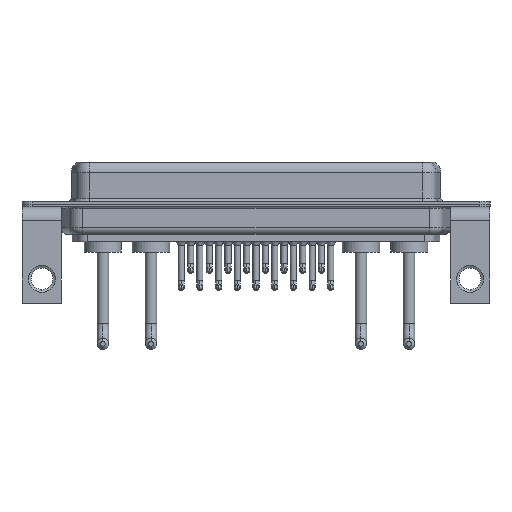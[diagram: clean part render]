
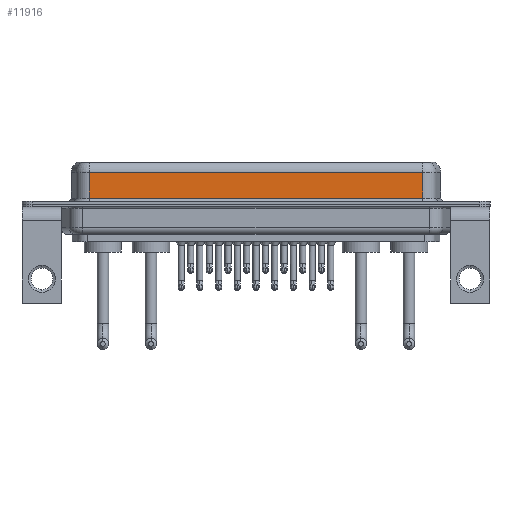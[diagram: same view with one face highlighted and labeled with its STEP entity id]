
A CAD part, front view. The second image highlights one B-rep face of the part: STEP entity #11916.
In plain terms, the highlighted planar face has unit normal (0, -1, 0).
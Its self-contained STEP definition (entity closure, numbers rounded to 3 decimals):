
#147 = EDGE_CURVE ( 'NONE', #21658, #11551, #12469, .T. ) ;
#1646 = CARTESIAN_POINT ( 'NONE',  ( 56.462, -3.95, 6.4 ) ) ;
#1962 = DIRECTION ( 'NONE',  ( 1., 0., 0. ) ) ;
#3037 = LINE ( 'NONE', #1646, #22165 ) ;
#3250 = VERTEX_POINT ( 'NONE', #12139 ) ;
#4416 = ORIENTED_EDGE ( 'NONE', *, *, #4469, .F. ) ;
#4469 = EDGE_CURVE ( 'NONE', #20727, #11551, #3037, .T. ) ;
#6838 = EDGE_CURVE ( 'NONE', #20727, #3250, #22439, .T. ) ;
#6859 = CARTESIAN_POINT ( 'NONE',  ( 56.462, -3.95, 6.4 ) ) ;
#7925 = ORIENTED_EDGE ( 'NONE', *, *, #147, .T. ) ;
#8530 = CARTESIAN_POINT ( 'NONE',  ( 7.038, -3.95, 6.4 ) ) ;
#10032 = ORIENTED_EDGE ( 'NONE', *, *, #20569, .T. ) ;
#10428 = DIRECTION ( 'NONE',  ( 0., 1., 0. ) ) ;
#10731 = CARTESIAN_POINT ( 'NONE',  ( 56.462, -3.95, 0.9 ) ) ;
#11551 = VERTEX_POINT ( 'NONE', #21988 ) ;
#11916 = ADVANCED_FACE ( 'NONE', ( #15606 ), #20798, .F. ) ;
#12139 = CARTESIAN_POINT ( 'NONE',  ( 7.038, -3.95, 4.65 ) ) ;
#12433 = VECTOR ( 'NONE', #1962, 1000. ) ;
#12469 = LINE ( 'NONE', #10731, #12433 ) ;
#12572 = ORIENTED_EDGE ( 'NONE', *, *, #6838, .T. ) ;
#13436 = VECTOR ( 'NONE', #15551, 1000. ) ;
#14943 = VECTOR ( 'NONE', #15079, 1000. ) ;
#15079 = DIRECTION ( 'NONE',  ( -1., 0., 0. ) ) ;
#15260 = DIRECTION ( 'NONE',  ( 0., 0., 1. ) ) ;
#15551 = DIRECTION ( 'NONE',  ( 0., 0., -1. ) ) ;
#15606 = FACE_OUTER_BOUND ( 'NONE', #17309, .T. ) ;
#17053 = CARTESIAN_POINT ( 'NONE',  ( 56.462, -3.95, 4.65 ) ) ;
#17309 = EDGE_LOOP ( 'NONE', ( #4416, #12572, #10032, #7925 ) ) ;
#18077 = CARTESIAN_POINT ( 'NONE',  ( 56.462, -3.95, 4.65 ) ) ;
#18350 = AXIS2_PLACEMENT_3D ( 'NONE', #6859, #10428, #15260 ) ;
#19015 = LINE ( 'NONE', #8530, #13436 ) ;
#20569 = EDGE_CURVE ( 'NONE', #3250, #21658, #19015, .T. ) ;
#20727 = VERTEX_POINT ( 'NONE', #18077 ) ;
#20798 = PLANE ( 'NONE',  #18350 ) ;
#20898 = DIRECTION ( 'NONE',  ( 0., 0., -1. ) ) ;
#21658 = VERTEX_POINT ( 'NONE', #22047 ) ;
#21988 = CARTESIAN_POINT ( 'NONE',  ( 56.462, -3.95, 0.9 ) ) ;
#22047 = CARTESIAN_POINT ( 'NONE',  ( 7.038, -3.95, 0.9 ) ) ;
#22165 = VECTOR ( 'NONE', #20898, 1000. ) ;
#22439 = LINE ( 'NONE', #17053, #14943 ) ;
